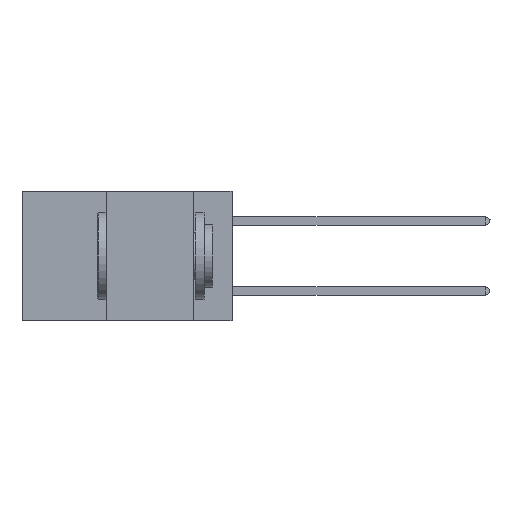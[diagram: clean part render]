
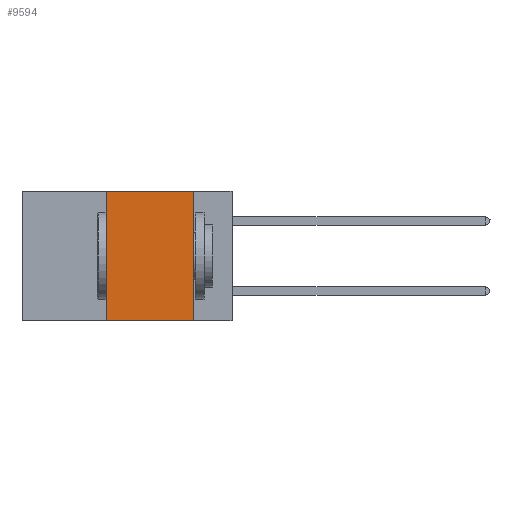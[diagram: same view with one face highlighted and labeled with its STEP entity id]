
A CAD part, left-side view. The second image highlights one B-rep face of the part: STEP entity #9594.
In plain terms, the highlighted planar face has unit normal (-1, 0, 0).
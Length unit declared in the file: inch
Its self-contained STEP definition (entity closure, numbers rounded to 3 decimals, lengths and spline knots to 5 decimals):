
#43 = CARTESIAN_POINT ( 'NONE',  ( 0., 0.11, 0. ) ) ;
#165 = CARTESIAN_POINT ( 'NONE',  ( 0., 0.36, 0. ) ) ;
#597 = VERTEX_POINT ( 'NONE', #12604 ) ;
#1365 = DIRECTION ( 'NONE',  ( 1., 0., 0. ) ) ;
#4459 = LINE ( 'NONE', #165, #12592 ) ;
#6416 = LINE ( 'NONE', #23861, #26819 ) ;
#8001 = CARTESIAN_POINT ( 'NONE',  ( 0., 0.11, -0.37 ) ) ;
#9242 = EDGE_CURVE ( 'NONE', #18992, #597, #4459, .T. ) ;
#9429 = CARTESIAN_POINT ( 'NONE',  ( 0., 0.6, 0. ) ) ;
#9594 = ADVANCED_FACE ( 'NONE', ( #15289 ), #27291, .F. ) ;
#9644 = ORIENTED_EDGE ( 'NONE', *, *, #9242, .F. ) ;
#9681 = DIRECTION ( 'NONE',  ( 0., -1., 0. ) ) ;
#10490 = DIRECTION ( 'NONE',  ( 0., 0., -1. ) ) ;
#12026 = LINE ( 'NONE', #9429, #12706 ) ;
#12165 = CARTESIAN_POINT ( 'NONE',  ( 0., 0.6, 0. ) ) ;
#12237 = VECTOR ( 'NONE', #9681, 39.37008 ) ;
#12592 = VECTOR ( 'NONE', #15325, 39.37008 ) ;
#12604 = CARTESIAN_POINT ( 'NONE',  ( 0., 0.36, 0. ) ) ;
#12706 = VECTOR ( 'NONE', #26531, 39.37008 ) ;
#13305 = ORIENTED_EDGE ( 'NONE', *, *, #22433, .T. ) ;
#13885 = AXIS2_PLACEMENT_3D ( 'NONE', #12165, #1365, #27379 ) ;
#14368 = VERTEX_POINT ( 'NONE', #8001 ) ;
#15289 = FACE_OUTER_BOUND ( 'NONE', #16312, .T. ) ;
#15325 = DIRECTION ( 'NONE',  ( 0., 0., 1. ) ) ;
#16312 = EDGE_LOOP ( 'NONE', ( #19337, #26586, #9644, #13305 ) ) ;
#18992 = VERTEX_POINT ( 'NONE', #27361 ) ;
#19337 = ORIENTED_EDGE ( 'NONE', *, *, #23482, .F. ) ;
#20685 = CARTESIAN_POINT ( 'NONE',  ( 0., 0.6, -0.37 ) ) ;
#22194 = VERTEX_POINT ( 'NONE', #43 ) ;
#22433 = EDGE_CURVE ( 'NONE', #18992, #14368, #24834, .T. ) ;
#23482 = EDGE_CURVE ( 'NONE', #22194, #14368, #6416, .T. ) ;
#23861 = CARTESIAN_POINT ( 'NONE',  ( 0., 0.11, 0. ) ) ;
#24834 = LINE ( 'NONE', #20685, #12237 ) ;
#26531 = DIRECTION ( 'NONE',  ( 0., -1., 0. ) ) ;
#26586 = ORIENTED_EDGE ( 'NONE', *, *, #26695, .F. ) ;
#26695 = EDGE_CURVE ( 'NONE', #597, #22194, #12026, .T. ) ;
#26819 = VECTOR ( 'NONE', #10490, 39.37008 ) ;
#27291 = PLANE ( 'NONE',  #13885 ) ;
#27361 = CARTESIAN_POINT ( 'NONE',  ( 0., 0.36, -0.37 ) ) ;
#27379 = DIRECTION ( 'NONE',  ( 0., 0., -1. ) ) ;
